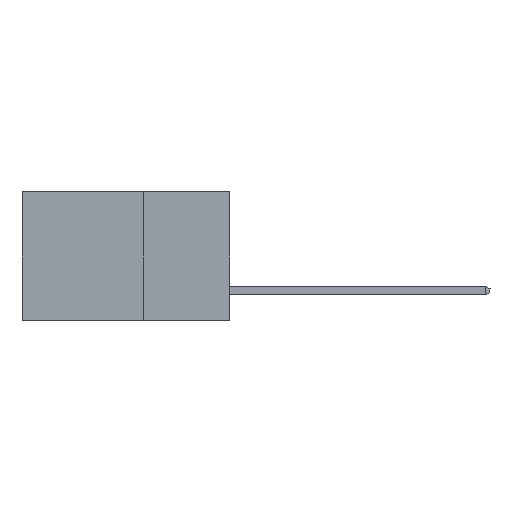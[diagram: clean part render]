
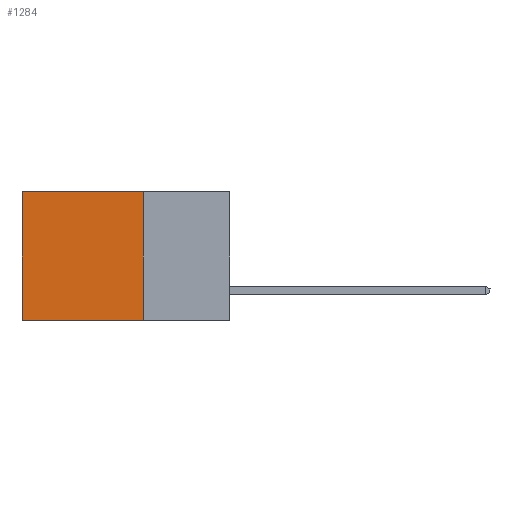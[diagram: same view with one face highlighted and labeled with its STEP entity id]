
A CAD part, left-side view. The second image highlights one B-rep face of the part: STEP entity #1284.
In plain terms, the highlighted planar face has unit normal (-1, 0, 0).
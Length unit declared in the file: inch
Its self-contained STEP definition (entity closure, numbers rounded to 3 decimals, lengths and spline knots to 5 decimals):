
#488 = CARTESIAN_POINT ( 'NONE',  ( 0.2615, 0.25, -0.37 ) ) ;
#1004 = PLANE ( 'NONE',  #12891 ) ;
#1127 = CARTESIAN_POINT ( 'NONE',  ( 0.2615, 0.25, -0.37 ) ) ;
#1284 = ADVANCED_FACE ( 'NONE', ( #18142 ), #1004, .F. ) ;
#2731 = EDGE_CURVE ( 'NONE', #8185, #13519, #22470, .T. ) ;
#3070 = ORIENTED_EDGE ( 'NONE', *, *, #2731, .T. ) ;
#4940 = DIRECTION ( 'NONE',  ( 0., 1., 0. ) ) ;
#5804 = EDGE_CURVE ( 'NONE', #13669, #10226, #13998, .T. ) ;
#6289 = ORIENTED_EDGE ( 'NONE', *, *, #15248, .F. ) ;
#6361 = DIRECTION ( 'NONE',  ( 0., 0., -1. ) ) ;
#7214 = CARTESIAN_POINT ( 'NONE',  ( 0.2615, 0.6, 0. ) ) ;
#7304 = LINE ( 'NONE', #12576, #10231 ) ;
#7983 = DIRECTION ( 'NONE',  ( 0., 0., -1. ) ) ;
#8185 = VERTEX_POINT ( 'NONE', #10804 ) ;
#9643 = EDGE_LOOP ( 'NONE', ( #22380, #13611, #6289, #3070 ) ) ;
#10226 = VERTEX_POINT ( 'NONE', #13424 ) ;
#10231 = VECTOR ( 'NONE', #14753, 39.37008 ) ;
#10325 = VECTOR ( 'NONE', #7983, 39.37008 ) ;
#10804 = CARTESIAN_POINT ( 'NONE',  ( 0.2615, 0.25, 0. ) ) ;
#11087 = LINE ( 'NONE', #488, #10325 ) ;
#12576 = CARTESIAN_POINT ( 'NONE',  ( 0.2615, 0.6, -0.37 ) ) ;
#12891 = AXIS2_PLACEMENT_3D ( 'NONE', #1127, #14647, #6361 ) ;
#13424 = CARTESIAN_POINT ( 'NONE',  ( 0.2615, 0.6, -0.37 ) ) ;
#13519 = VERTEX_POINT ( 'NONE', #7214 ) ;
#13611 = ORIENTED_EDGE ( 'NONE', *, *, #5804, .F. ) ;
#13669 = VERTEX_POINT ( 'NONE', #16435 ) ;
#13998 = LINE ( 'NONE', #20956, #21196 ) ;
#14555 = VECTOR ( 'NONE', #19109, 39.37008 ) ;
#14647 = DIRECTION ( 'NONE',  ( 1., 0., 0. ) ) ;
#14753 = DIRECTION ( 'NONE',  ( 0., 0., -1. ) ) ;
#15248 = EDGE_CURVE ( 'NONE', #8185, #13669, #11087, .T. ) ;
#16435 = CARTESIAN_POINT ( 'NONE',  ( 0.2615, 0.25, -0.37 ) ) ;
#18142 = FACE_OUTER_BOUND ( 'NONE', #9643, .T. ) ;
#19014 = EDGE_CURVE ( 'NONE', #13519, #10226, #7304, .T. ) ;
#19109 = DIRECTION ( 'NONE',  ( 0., 1., 0. ) ) ;
#20956 = CARTESIAN_POINT ( 'NONE',  ( 0.2615, 0.25, -0.37 ) ) ;
#21196 = VECTOR ( 'NONE', #4940, 39.37008 ) ;
#22359 = CARTESIAN_POINT ( 'NONE',  ( 0.2615, 0.25, 0. ) ) ;
#22380 = ORIENTED_EDGE ( 'NONE', *, *, #19014, .T. ) ;
#22470 = LINE ( 'NONE', #22359, #14555 ) ;
